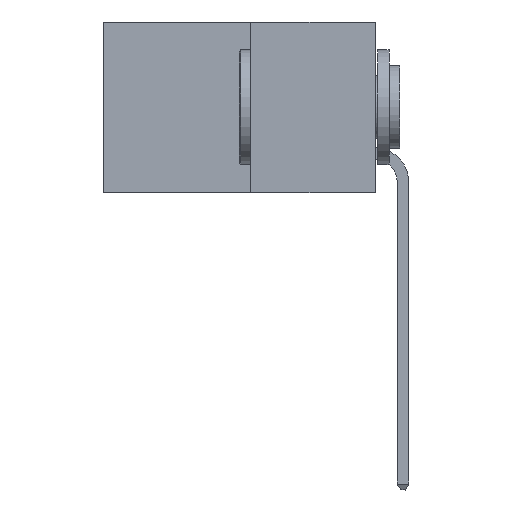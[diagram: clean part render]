
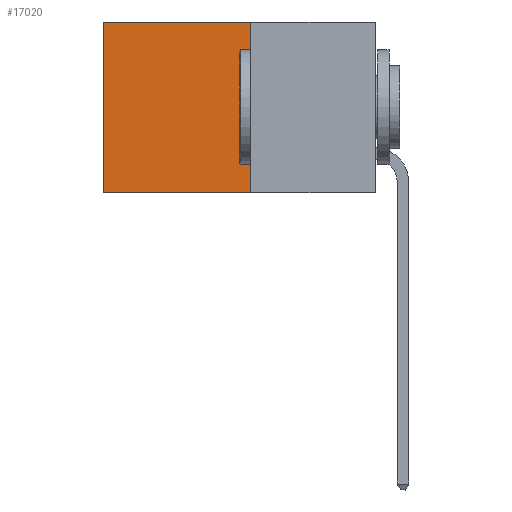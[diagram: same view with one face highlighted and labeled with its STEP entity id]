
A CAD part, left-side view. The second image highlights one B-rep face of the part: STEP entity #17020.
In plain terms, the highlighted planar face has unit normal (-1, 0, 0).
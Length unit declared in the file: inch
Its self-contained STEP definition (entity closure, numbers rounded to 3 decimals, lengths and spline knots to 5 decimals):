
#176 = VERTEX_POINT ( 'NONE', #17651 ) ;
#320 = VERTEX_POINT ( 'NONE', #21179 ) ;
#1064 = DIRECTION ( 'NONE',  ( 1., 0., 0. ) ) ;
#1724 = LINE ( 'NONE', #23568, #26614 ) ;
#3785 = DIRECTION ( 'NONE',  ( 0., 1., 0. ) ) ;
#5408 = AXIS2_PLACEMENT_3D ( 'NONE', #15652, #1064, #18086 ) ;
#5738 = ORIENTED_EDGE ( 'NONE', *, *, #29393, .T. ) ;
#6163 = EDGE_CURVE ( 'NONE', #14293, #176, #1724, .T. ) ;
#6539 = ORIENTED_EDGE ( 'NONE', *, *, #21433, .F. ) ;
#8629 = ORIENTED_EDGE ( 'NONE', *, *, #6163, .F. ) ;
#8907 = VECTOR ( 'NONE', #20325, 39.37008 ) ;
#9028 = ORIENTED_EDGE ( 'NONE', *, *, #22607, .T. ) ;
#10129 = DIRECTION ( 'NONE',  ( 0., 0., -1. ) ) ;
#10234 = VERTEX_POINT ( 'NONE', #22599 ) ;
#10317 = LINE ( 'NONE', #11062, #17518 ) ;
#11062 = CARTESIAN_POINT ( 'NONE',  ( 0.277, 0.27, 0. ) ) ;
#12550 = CARTESIAN_POINT ( 'NONE',  ( 0.277, 0.27, 0. ) ) ;
#13023 = CARTESIAN_POINT ( 'NONE',  ( 0.277, 0.27, -0.37 ) ) ;
#14293 = VERTEX_POINT ( 'NONE', #12550 ) ;
#14877 = LINE ( 'NONE', #17420, #26817 ) ;
#15323 = LINE ( 'NONE', #13023, #8907 ) ;
#15652 = CARTESIAN_POINT ( 'NONE',  ( 0.277, 0.27, -0.37 ) ) ;
#17020 = ADVANCED_FACE ( 'NONE', ( #26355 ), #25143, .F. ) ;
#17420 = CARTESIAN_POINT ( 'NONE',  ( 0.277, 0.59, -0.37 ) ) ;
#17518 = VECTOR ( 'NONE', #3785, 39.37008 ) ;
#17651 = CARTESIAN_POINT ( 'NONE',  ( 0.277, 0.27, -0.37 ) ) ;
#18086 = DIRECTION ( 'NONE',  ( 0., 0., -1. ) ) ;
#20325 = DIRECTION ( 'NONE',  ( 0., 1., 0. ) ) ;
#21179 = CARTESIAN_POINT ( 'NONE',  ( 0.277, 0.59, -0.37 ) ) ;
#21294 = EDGE_LOOP ( 'NONE', ( #5738, #6539, #8629, #9028 ) ) ;
#21433 = EDGE_CURVE ( 'NONE', #176, #320, #15323, .T. ) ;
#22599 = CARTESIAN_POINT ( 'NONE',  ( 0.277, 0.59, 0. ) ) ;
#22607 = EDGE_CURVE ( 'NONE', #14293, #10234, #10317, .T. ) ;
#23321 = DIRECTION ( 'NONE',  ( 0., 0., -1. ) ) ;
#23568 = CARTESIAN_POINT ( 'NONE',  ( 0.277, 0.27, -0.37 ) ) ;
#25143 = PLANE ( 'NONE',  #5408 ) ;
#26355 = FACE_OUTER_BOUND ( 'NONE', #21294, .T. ) ;
#26614 = VECTOR ( 'NONE', #23321, 39.37008 ) ;
#26817 = VECTOR ( 'NONE', #10129, 39.37008 ) ;
#29393 = EDGE_CURVE ( 'NONE', #10234, #320, #14877, .T. ) ;
